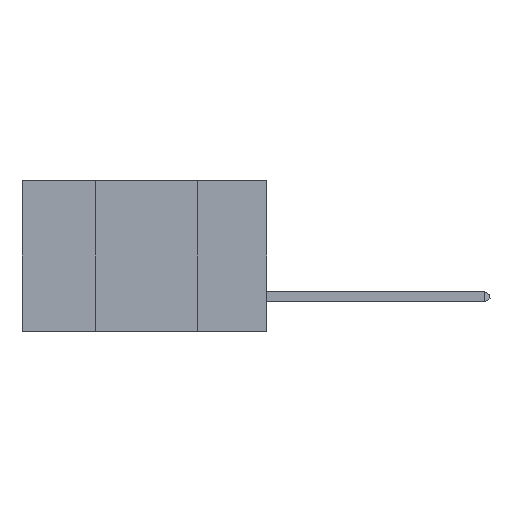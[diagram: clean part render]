
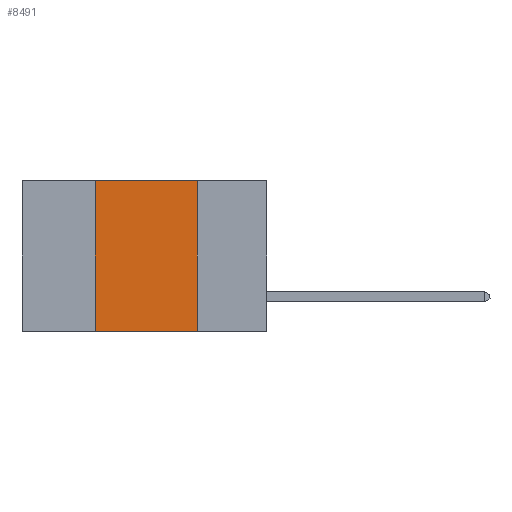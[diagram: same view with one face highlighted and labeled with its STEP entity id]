
A CAD part, left-side view. The second image highlights one B-rep face of the part: STEP entity #8491.
In plain terms, the highlighted planar face has unit normal (-1, 0, 0).
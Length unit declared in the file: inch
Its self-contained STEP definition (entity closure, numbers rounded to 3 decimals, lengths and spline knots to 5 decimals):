
#292 = CARTESIAN_POINT ( 'NONE',  ( 0., 0.6, 0. ) ) ;
#1987 = PLANE ( 'NONE',  #16953 ) ;
#2550 = CARTESIAN_POINT ( 'NONE',  ( 0., 0.17, 0. ) ) ;
#2654 = ORIENTED_EDGE ( 'NONE', *, *, #11919, .F. ) ;
#2899 = VECTOR ( 'NONE', #17508, 39.37008 ) ;
#3629 = DIRECTION ( 'NONE',  ( 1., 0., 0. ) ) ;
#4277 = CARTESIAN_POINT ( 'NONE',  ( 0., 0.6, -0.37 ) ) ;
#5905 = DIRECTION ( 'NONE',  ( 0., -1., 0. ) ) ;
#6760 = EDGE_CURVE ( 'NONE', #13907, #9641, #18370, .T. ) ;
#6819 = CARTESIAN_POINT ( 'NONE',  ( 0., 0.42, -0.37 ) ) ;
#6935 = ORIENTED_EDGE ( 'NONE', *, *, #17295, .F. ) ;
#7229 = FACE_OUTER_BOUND ( 'NONE', #11430, .T. ) ;
#7252 = VERTEX_POINT ( 'NONE', #17175 ) ;
#7411 = ORIENTED_EDGE ( 'NONE', *, *, #14299, .T. ) ;
#8491 = ADVANCED_FACE ( 'NONE', ( #7229 ), #1987, .F. ) ;
#9641 = VERTEX_POINT ( 'NONE', #12528 ) ;
#10448 = DIRECTION ( 'NONE',  ( 0., 0., -1. ) ) ;
#11157 = VECTOR ( 'NONE', #5905, 39.37008 ) ;
#11299 = LINE ( 'NONE', #16045, #2899 ) ;
#11430 = EDGE_LOOP ( 'NONE', ( #14572, #2654, #6935, #7411 ) ) ;
#11620 = LINE ( 'NONE', #4277, #11157 ) ;
#11919 = EDGE_CURVE ( 'NONE', #7252, #13907, #13825, .T. ) ;
#12528 = CARTESIAN_POINT ( 'NONE',  ( 0., 0.17, -0.37 ) ) ;
#12600 = CARTESIAN_POINT ( 'NONE',  ( 0., 0.17, 0. ) ) ;
#13825 = LINE ( 'NONE', #16920, #14297 ) ;
#13907 = VERTEX_POINT ( 'NONE', #12600 ) ;
#13931 = DIRECTION ( 'NONE',  ( 0., -1., 0. ) ) ;
#14297 = VECTOR ( 'NONE', #13931, 39.37008 ) ;
#14299 = EDGE_CURVE ( 'NONE', #19942, #9641, #11620, .T. ) ;
#14460 = VECTOR ( 'NONE', #10448, 39.37008 ) ;
#14466 = DIRECTION ( 'NONE',  ( 0., 0., -1. ) ) ;
#14572 = ORIENTED_EDGE ( 'NONE', *, *, #6760, .F. ) ;
#16045 = CARTESIAN_POINT ( 'NONE',  ( 0., 0.42, 0. ) ) ;
#16920 = CARTESIAN_POINT ( 'NONE',  ( 0., 0.6, 0. ) ) ;
#16953 = AXIS2_PLACEMENT_3D ( 'NONE', #292, #3629, #14466 ) ;
#17175 = CARTESIAN_POINT ( 'NONE',  ( 0., 0.42, 0. ) ) ;
#17295 = EDGE_CURVE ( 'NONE', #19942, #7252, #11299, .T. ) ;
#17508 = DIRECTION ( 'NONE',  ( 0., 0., 1. ) ) ;
#18370 = LINE ( 'NONE', #2550, #14460 ) ;
#19942 = VERTEX_POINT ( 'NONE', #6819 ) ;
